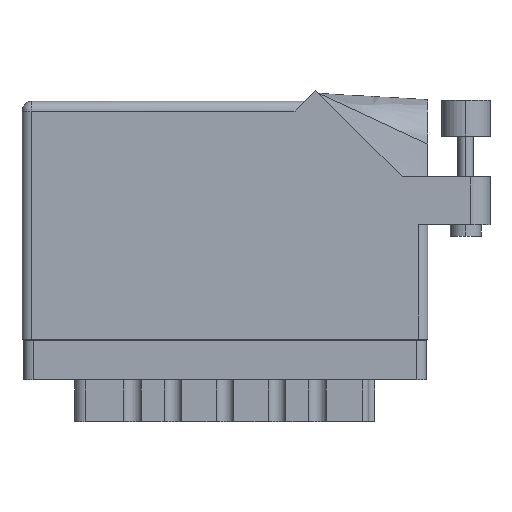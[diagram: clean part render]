
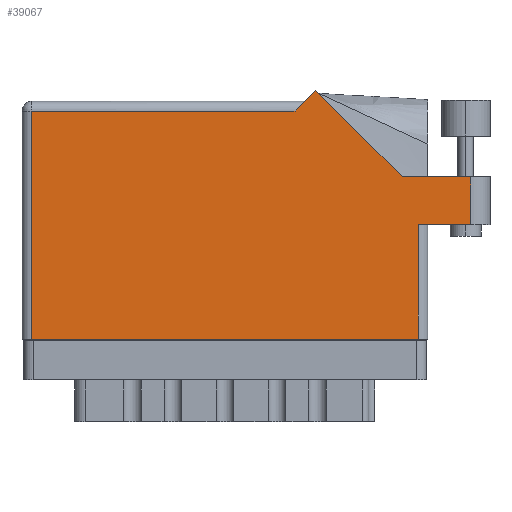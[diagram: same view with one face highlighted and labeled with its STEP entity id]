
A CAD part, front view. The second image highlights one B-rep face of the part: STEP entity #39067.
In plain terms, the highlighted face is planar.
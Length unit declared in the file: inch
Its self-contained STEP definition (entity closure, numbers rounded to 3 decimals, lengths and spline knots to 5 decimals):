
#71 = CARTESIAN_POINT ( 'NONE',  ( 2.44642, 1.044, 0. ) ) ;
#408 = CARTESIAN_POINT ( 'NONE',  ( 2.887, 1.044, 0. ) ) ;
#927 = EDGE_LOOP ( 'NONE', ( #48355, #15874, #30621, #40889, #26313, #22123, #11336, #24613, #9947 ) ) ;
#1747 = CARTESIAN_POINT ( 'NONE',  ( 0., 1.468, 0. ) ) ;
#2328 = CARTESIAN_POINT ( 'NONE',  ( 2.55, 0.737, 0. ) ) ;
#3592 = VECTOR ( 'NONE', #49041, 39.37008 ) ;
#5309 = CARTESIAN_POINT ( 'NONE',  ( 1.757, 1.468, 0. ) ) ;
#6711 = CARTESIAN_POINT ( 'NONE',  ( 0., 0., 0. ) ) ;
#7038 = CARTESIAN_POINT ( 'NONE',  ( 0.062, 0., 0. ) ) ;
#7341 = EDGE_CURVE ( 'NONE', #22766, #42427, #31884, .T. ) ;
#7560 = VECTOR ( 'NONE', #24998, 39.37008 ) ;
#7653 = LINE ( 'NONE', #1747, #39477 ) ;
#8299 = VERTEX_POINT ( 'NONE', #7038 ) ;
#9035 = VERTEX_POINT ( 'NONE', #40644 ) ;
#9478 = CARTESIAN_POINT ( 'NONE',  ( 2.55, 0.737, 0. ) ) ;
#9947 = ORIENTED_EDGE ( 'NONE', *, *, #30268, .T. ) ;
#9996 = DIRECTION ( 'NONE',  ( 0., 1., 0. ) ) ;
#10122 = LINE ( 'NONE', #44664, #3592 ) ;
#10304 = VERTEX_POINT ( 'NONE', #24864 ) ;
#11336 = ORIENTED_EDGE ( 'NONE', *, *, #41009, .T. ) ;
#11610 = LINE ( 'NONE', #33404, #41036 ) ;
#11967 = VECTOR ( 'NONE', #13547, 39.37008 ) ;
#13281 = DIRECTION ( 'NONE',  ( -1., 0., 0. ) ) ;
#13547 = DIRECTION ( 'NONE',  ( 0., -1., 0. ) ) ;
#15454 = VECTOR ( 'NONE', #9996, 39.37008 ) ;
#15874 = ORIENTED_EDGE ( 'NONE', *, *, #34325, .T. ) ;
#19653 = LINE ( 'NONE', #2328, #15454 ) ;
#21060 = DIRECTION ( 'NONE',  ( 0., 0., -1. ) ) ;
#21659 = DIRECTION ( 'NONE',  ( 1., 0., 0. ) ) ;
#22123 = ORIENTED_EDGE ( 'NONE', *, *, #48399, .T. ) ;
#22225 = CARTESIAN_POINT ( 'NONE',  ( 2.44642, 1.044, 0. ) ) ;
#22766 = VERTEX_POINT ( 'NONE', #71 ) ;
#23443 = VECTOR ( 'NONE', #41864, 39.37008 ) ;
#24103 = VECTOR ( 'NONE', #26387, 39.37008 ) ;
#24525 = CARTESIAN_POINT ( 'NONE',  ( 1.819, 1.53, 0. ) ) ;
#24613 = ORIENTED_EDGE ( 'NONE', *, *, #43568, .T. ) ;
#24864 = CARTESIAN_POINT ( 'NONE',  ( 2.55, 0., 0. ) ) ;
#24998 = DIRECTION ( 'NONE',  ( -0.707, -0.707, 0. ) ) ;
#25551 = CARTESIAN_POINT ( 'NONE',  ( 0., 1.53, 0. ) ) ;
#26313 = ORIENTED_EDGE ( 'NONE', *, *, #43449, .T. ) ;
#26387 = DIRECTION ( 'NONE',  ( -0.707, 0.707, 0. ) ) ;
#26729 = LINE ( 'NONE', #24525, #7560 ) ;
#26840 = EDGE_CURVE ( 'NONE', #44727, #22766, #11610, .T. ) ;
#27542 = LINE ( 'NONE', #36549, #11967 ) ;
#28741 = DIRECTION ( 'NONE',  ( -1., 0., 0. ) ) ;
#30268 = EDGE_CURVE ( 'NONE', #10304, #33385, #19653, .T. ) ;
#30621 = ORIENTED_EDGE ( 'NONE', *, *, #26840, .T. ) ;
#31031 = AXIS2_PLACEMENT_3D ( 'NONE', #25551, #21060, #28741 ) ;
#31884 = LINE ( 'NONE', #22225, #24103 ) ;
#33385 = VERTEX_POINT ( 'NONE', #9478 ) ;
#33404 = CARTESIAN_POINT ( 'NONE',  ( 3.012, 1.044, 0. ) ) ;
#34325 = EDGE_CURVE ( 'NONE', #9035, #44727, #36635, .T. ) ;
#35016 = VERTEX_POINT ( 'NONE', #43245 ) ;
#35099 = VERTEX_POINT ( 'NONE', #5309 ) ;
#35508 = FACE_OUTER_BOUND ( 'NONE', #927, .T. ) ;
#36549 = CARTESIAN_POINT ( 'NONE',  ( 0.062, 0., 0. ) ) ;
#36635 = LINE ( 'NONE', #38007, #23443 ) ;
#37105 = DIRECTION ( 'NONE',  ( -1., 0., 0. ) ) ;
#38007 = CARTESIAN_POINT ( 'NONE',  ( 2.887, 1.044, 0. ) ) ;
#39067 = ADVANCED_FACE ( 'NONE', ( #35508 ), #44053, .F. ) ;
#39386 = LINE ( 'NONE', #6711, #46625 ) ;
#39477 = VECTOR ( 'NONE', #13281, 39.37008 ) ;
#40644 = CARTESIAN_POINT ( 'NONE',  ( 2.887, 0.737, 0. ) ) ;
#40889 = ORIENTED_EDGE ( 'NONE', *, *, #7341, .T. ) ;
#41009 = EDGE_CURVE ( 'NONE', #35016, #8299, #27542, .T. ) ;
#41036 = VECTOR ( 'NONE', #37105, 39.37008 ) ;
#41864 = DIRECTION ( 'NONE',  ( 0., 1., 0. ) ) ;
#42427 = VERTEX_POINT ( 'NONE', #49410 ) ;
#43245 = CARTESIAN_POINT ( 'NONE',  ( 0.062, 1.468, 0. ) ) ;
#43449 = EDGE_CURVE ( 'NONE', #42427, #35099, #26729, .T. ) ;
#43568 = EDGE_CURVE ( 'NONE', #8299, #10304, #39386, .T. ) ;
#44053 = PLANE ( 'NONE',  #31031 ) ;
#44664 = CARTESIAN_POINT ( 'NONE',  ( 2.612, 0.737, 0. ) ) ;
#44727 = VERTEX_POINT ( 'NONE', #408 ) ;
#46625 = VECTOR ( 'NONE', #21659, 39.37008 ) ;
#46826 = EDGE_CURVE ( 'NONE', #33385, #9035, #10122, .T. ) ;
#48355 = ORIENTED_EDGE ( 'NONE', *, *, #46826, .T. ) ;
#48399 = EDGE_CURVE ( 'NONE', #35099, #35016, #7653, .T. ) ;
#49041 = DIRECTION ( 'NONE',  ( 1., 0., 0. ) ) ;
#49410 = CARTESIAN_POINT ( 'NONE',  ( 1.88971, 1.60071, 0. ) ) ;
